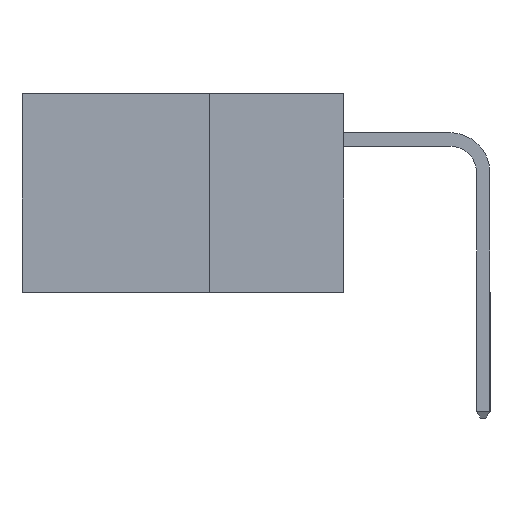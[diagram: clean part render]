
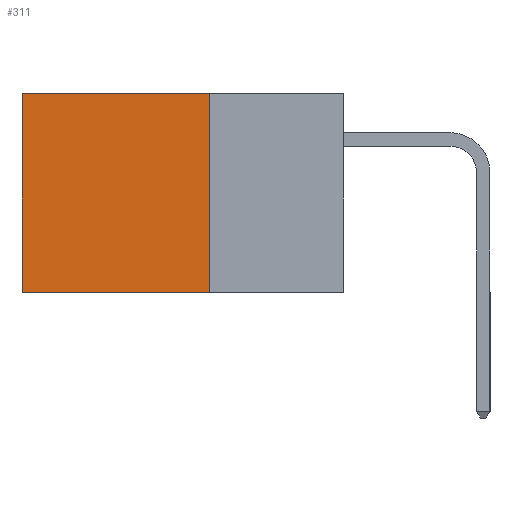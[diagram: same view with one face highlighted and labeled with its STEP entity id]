
A CAD part, left-side view. The second image highlights one B-rep face of the part: STEP entity #311.
In plain terms, the highlighted planar face has unit normal (-1, 0, 0).
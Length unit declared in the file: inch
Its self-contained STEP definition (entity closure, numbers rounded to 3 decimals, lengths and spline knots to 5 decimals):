
#147 = DIRECTION ( 'NONE',  ( 1., 0., 0. ) ) ;
#263 = CARTESIAN_POINT ( 'NONE',  ( 0.298, 0.6, 0. ) ) ;
#311 = ADVANCED_FACE ( 'NONE', ( #10087 ), #6919, .F. ) ;
#877 = ORIENTED_EDGE ( 'NONE', *, *, #4727, .T. ) ;
#981 = CARTESIAN_POINT ( 'NONE',  ( 0.298, 0.25, 0. ) ) ;
#2080 = ORIENTED_EDGE ( 'NONE', *, *, #9498, .F. ) ;
#2743 = VERTEX_POINT ( 'NONE', #8493 ) ;
#2886 = VECTOR ( 'NONE', #6597, 39.37008 ) ;
#3171 = EDGE_CURVE ( 'NONE', #2743, #4054, #5192, .T. ) ;
#3636 = CARTESIAN_POINT ( 'NONE',  ( 0.298, 0.25, -0.37 ) ) ;
#3754 = LINE ( 'NONE', #981, #6115 ) ;
#3959 = VERTEX_POINT ( 'NONE', #7845 ) ;
#4054 = VERTEX_POINT ( 'NONE', #4734 ) ;
#4727 = EDGE_CURVE ( 'NONE', #3959, #4054, #5292, .T. ) ;
#4734 = CARTESIAN_POINT ( 'NONE',  ( 0.298, 0.6, -0.37 ) ) ;
#5168 = EDGE_CURVE ( 'NONE', #10281, #3959, #3754, .T. ) ;
#5192 = LINE ( 'NONE', #3636, #8428 ) ;
#5292 = LINE ( 'NONE', #263, #2886 ) ;
#5549 = EDGE_LOOP ( 'NONE', ( #877, #10950, #2080, #10393 ) ) ;
#6115 = VECTOR ( 'NONE', #6392, 39.37008 ) ;
#6392 = DIRECTION ( 'NONE',  ( 0., 1., 0. ) ) ;
#6443 = CARTESIAN_POINT ( 'NONE',  ( 0.298, 0.25, 0. ) ) ;
#6597 = DIRECTION ( 'NONE',  ( 0., 0., -1. ) ) ;
#6910 = CARTESIAN_POINT ( 'NONE',  ( 0.298, 0.25, 0. ) ) ;
#6919 = PLANE ( 'NONE',  #10261 ) ;
#7032 = DIRECTION ( 'NONE',  ( 0., 0., -1. ) ) ;
#7828 = VECTOR ( 'NONE', #7032, 39.37008 ) ;
#7845 = CARTESIAN_POINT ( 'NONE',  ( 0.298, 0.6, 0. ) ) ;
#8428 = VECTOR ( 'NONE', #10986, 39.37008 ) ;
#8493 = CARTESIAN_POINT ( 'NONE',  ( 0.298, 0.25, -0.37 ) ) ;
#9306 = CARTESIAN_POINT ( 'NONE',  ( 0.298, 0.25, 0. ) ) ;
#9498 = EDGE_CURVE ( 'NONE', #10281, #2743, #9913, .T. ) ;
#9913 = LINE ( 'NONE', #9306, #7828 ) ;
#10087 = FACE_OUTER_BOUND ( 'NONE', #5549, .T. ) ;
#10236 = DIRECTION ( 'NONE',  ( 0., 0., -1. ) ) ;
#10261 = AXIS2_PLACEMENT_3D ( 'NONE', #6910, #147, #10236 ) ;
#10281 = VERTEX_POINT ( 'NONE', #6443 ) ;
#10393 = ORIENTED_EDGE ( 'NONE', *, *, #5168, .T. ) ;
#10950 = ORIENTED_EDGE ( 'NONE', *, *, #3171, .F. ) ;
#10986 = DIRECTION ( 'NONE',  ( 0., 1., 0. ) ) ;
